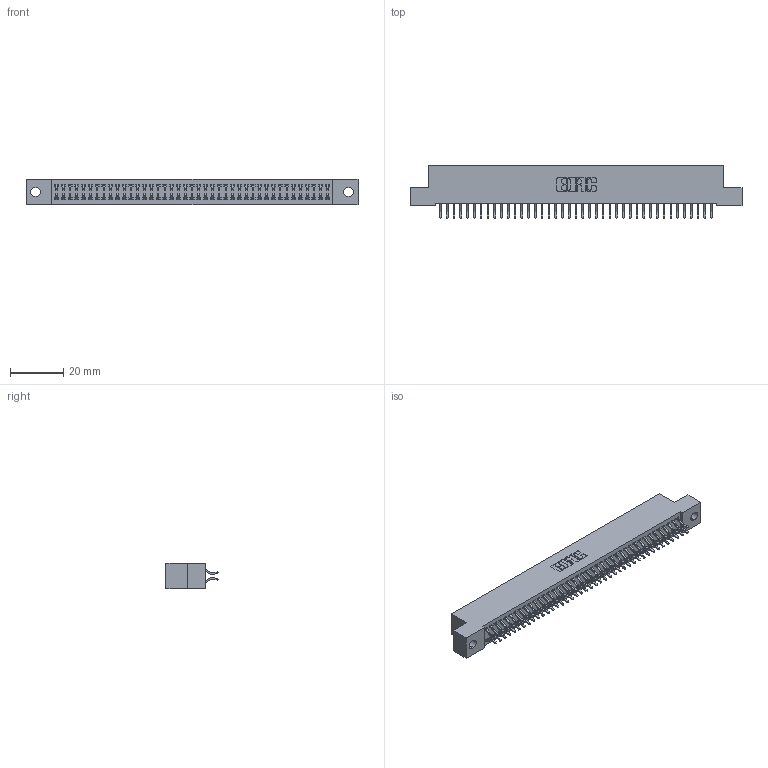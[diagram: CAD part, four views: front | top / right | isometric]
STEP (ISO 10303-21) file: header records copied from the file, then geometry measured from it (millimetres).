
FILE_DESCRIPTION (( 'STEP AP203' ), '1' );
FILE_NAME ('392-082-556-202.STEP', '2019-10-09T15:15:11', ( '' ), ( '' ), 'SwSTEP 2.0', 'SolidWorks 2016', '' );
FILE_SCHEMA (( 'CONFIG_CONTROL_DESIGN' ));
Length unit declared in the file: inch
Products named in the file (3): 342 Part_.128 Slot; 345-292-001_556 Tail; 392-082-556-202
Assembly tree (83 placements, depth 2):
  392-082-556-202
    342 Part_.128 Slot
    345-292-001_556 Tail  x82
Bounding box: 124.46 x 19.58 x 9.4 mm (x, y, z)
Volume: 11123.8 mm3; surface area: 17762 mm2
Topology: 83 solids, 83 shells, 4870 faces, 14497 edges, 9554 vertices
Faces by surface type: plane 3350, cylinder 1520
Entity records: 26729 total; most frequent: CARTESIAN_POINT 4446, ORIENTED_EDGE 4370, DIRECTION 3789, EDGE_CURVE 2185, VECTOR 2049, LINE 2049, VERTEX_POINT 1454, AXIS2_PLACEMENT_3D 870
